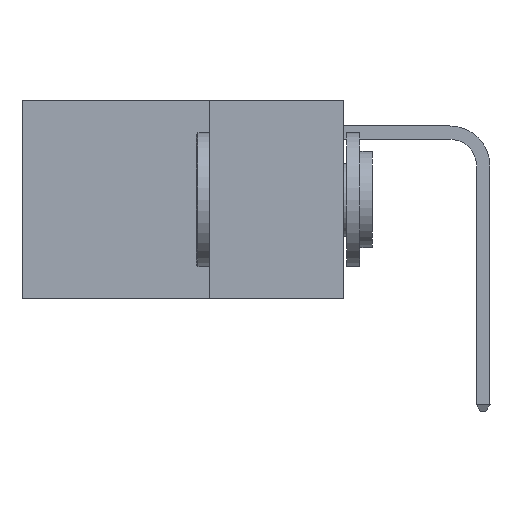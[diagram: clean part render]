
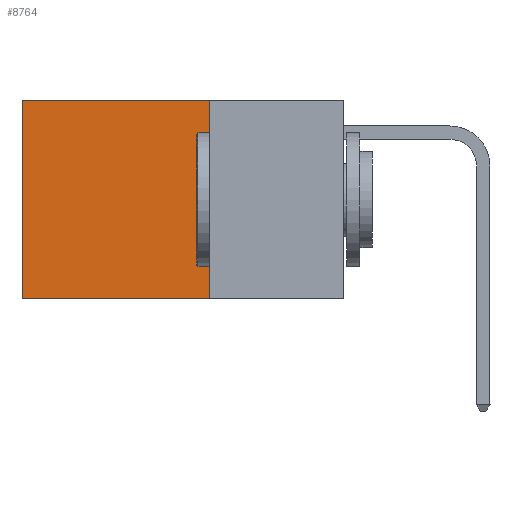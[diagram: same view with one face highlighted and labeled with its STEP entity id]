
A CAD part, left-side view. The second image highlights one B-rep face of the part: STEP entity #8764.
In plain terms, the highlighted planar face has unit normal (-1, 0, 0).
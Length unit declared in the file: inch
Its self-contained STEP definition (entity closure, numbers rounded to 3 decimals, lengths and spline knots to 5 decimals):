
#504 = ORIENTED_EDGE ( 'NONE', *, *, #778, .T. ) ;
#765 = EDGE_CURVE ( 'NONE', #5641, #10286, #14272, .T. ) ;
#778 = EDGE_CURVE ( 'NONE', #5129, #10286, #3600, .T. ) ;
#1484 = LINE ( 'NONE', #2835, #4278 ) ;
#2835 = CARTESIAN_POINT ( 'NONE',  ( 0.2625, 0.25, 0. ) ) ;
#3600 = LINE ( 'NONE', #7319, #4770 ) ;
#3727 = LINE ( 'NONE', #6075, #6074 ) ;
#3737 = EDGE_CURVE ( 'NONE', #3990, #5641, #3727, .T. ) ;
#3990 = VERTEX_POINT ( 'NONE', #7525 ) ;
#4218 = CARTESIAN_POINT ( 'NONE',  ( 0.2625, 0.25, -0.37 ) ) ;
#4278 = VECTOR ( 'NONE', #5125, 39.37008 ) ;
#4662 = EDGE_LOOP ( 'NONE', ( #504, #5696, #8650, #9316 ) ) ;
#4713 = PLANE ( 'NONE',  #12611 ) ;
#4770 = VECTOR ( 'NONE', #8322, 39.37008 ) ;
#5125 = DIRECTION ( 'NONE',  ( 0., 1., 0. ) ) ;
#5129 = VERTEX_POINT ( 'NONE', #14112 ) ;
#5641 = VERTEX_POINT ( 'NONE', #4218 ) ;
#5696 = ORIENTED_EDGE ( 'NONE', *, *, #765, .F. ) ;
#6074 = VECTOR ( 'NONE', #10691, 39.37008 ) ;
#6075 = CARTESIAN_POINT ( 'NONE',  ( 0.2625, 0.25, 0. ) ) ;
#6928 = FACE_OUTER_BOUND ( 'NONE', #4662, .T. ) ;
#7319 = CARTESIAN_POINT ( 'NONE',  ( 0.2625, 0.6, 0. ) ) ;
#7525 = CARTESIAN_POINT ( 'NONE',  ( 0.2625, 0.25, 0. ) ) ;
#8233 = DIRECTION ( 'NONE',  ( 0., 0., -1. ) ) ;
#8322 = DIRECTION ( 'NONE',  ( 0., 0., -1. ) ) ;
#8650 = ORIENTED_EDGE ( 'NONE', *, *, #3737, .F. ) ;
#8677 = VECTOR ( 'NONE', #11806, 39.37008 ) ;
#8764 = ADVANCED_FACE ( 'NONE', ( #6928 ), #4713, .F. ) ;
#9316 = ORIENTED_EDGE ( 'NONE', *, *, #11609, .T. ) ;
#9376 = CARTESIAN_POINT ( 'NONE',  ( 0.2625, 0.25, 0. ) ) ;
#10286 = VERTEX_POINT ( 'NONE', #11357 ) ;
#10691 = DIRECTION ( 'NONE',  ( 0., 0., -1. ) ) ;
#11357 = CARTESIAN_POINT ( 'NONE',  ( 0.2625, 0.6, -0.37 ) ) ;
#11609 = EDGE_CURVE ( 'NONE', #3990, #5129, #1484, .T. ) ;
#11806 = DIRECTION ( 'NONE',  ( 0., 1., 0. ) ) ;
#12611 = AXIS2_PLACEMENT_3D ( 'NONE', #9376, #14033, #8233 ) ;
#14033 = DIRECTION ( 'NONE',  ( 1., 0., 0. ) ) ;
#14112 = CARTESIAN_POINT ( 'NONE',  ( 0.2625, 0.6, 0. ) ) ;
#14188 = CARTESIAN_POINT ( 'NONE',  ( 0.2625, 0.25, -0.37 ) ) ;
#14272 = LINE ( 'NONE', #14188, #8677 ) ;
